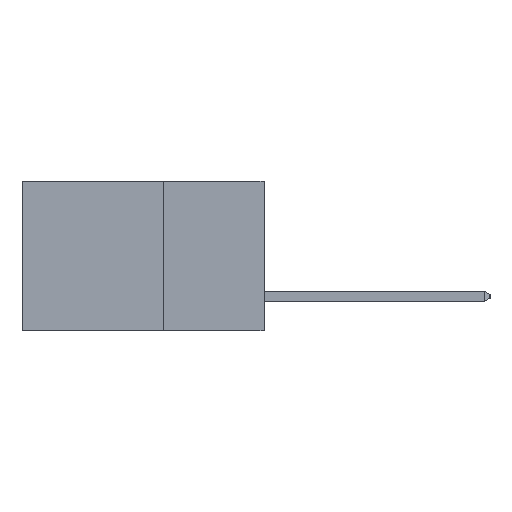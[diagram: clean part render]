
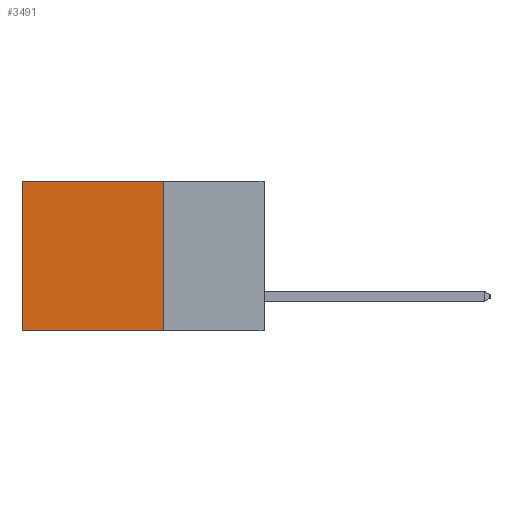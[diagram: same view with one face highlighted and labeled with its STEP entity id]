
A CAD part, left-side view. The second image highlights one B-rep face of the part: STEP entity #3491.
In plain terms, the highlighted planar face has unit normal (-1, 0, 0).
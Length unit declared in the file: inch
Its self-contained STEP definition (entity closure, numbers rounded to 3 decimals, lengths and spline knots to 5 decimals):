
#168 = EDGE_CURVE ( 'NONE', #5273, #9356, #3385, .T. ) ;
#925 = LINE ( 'NONE', #4226, #9724 ) ;
#1119 = DIRECTION ( 'NONE',  ( 0., 0., -1. ) ) ;
#1167 = DIRECTION ( 'NONE',  ( 1., 0., 0. ) ) ;
#1195 = CARTESIAN_POINT ( 'NONE',  ( 0.2615, 0.25, -0.37 ) ) ;
#1215 = PLANE ( 'NONE',  #4632 ) ;
#1447 = DIRECTION ( 'NONE',  ( 0., 1., 0. ) ) ;
#1473 = CARTESIAN_POINT ( 'NONE',  ( 0.2615, 0.25, -0.37 ) ) ;
#1525 = EDGE_CURVE ( 'NONE', #9356, #10380, #7017, .T. ) ;
#2842 = DIRECTION ( 'NONE',  ( 0., 1., 0. ) ) ;
#3385 = LINE ( 'NONE', #4524, #9996 ) ;
#3491 = ADVANCED_FACE ( 'NONE', ( #5857 ), #1215, .F. ) ;
#3927 = VECTOR ( 'NONE', #2842, 39.37008 ) ;
#4226 = CARTESIAN_POINT ( 'NONE',  ( 0.2615, 0.6, -0.37 ) ) ;
#4477 = VECTOR ( 'NONE', #1447, 39.37008 ) ;
#4524 = CARTESIAN_POINT ( 'NONE',  ( 0.2615, 0.25, -0.37 ) ) ;
#4539 = DIRECTION ( 'NONE',  ( 0., 0., -1. ) ) ;
#4632 = AXIS2_PLACEMENT_3D ( 'NONE', #1195, #1167, #1119 ) ;
#5273 = VERTEX_POINT ( 'NONE', #5674 ) ;
#5674 = CARTESIAN_POINT ( 'NONE',  ( 0.2615, 0.25, 0. ) ) ;
#5857 = FACE_OUTER_BOUND ( 'NONE', #10100, .T. ) ;
#6485 = ORIENTED_EDGE ( 'NONE', *, *, #9236, .T. ) ;
#6645 = ORIENTED_EDGE ( 'NONE', *, *, #8902, .T. ) ;
#6805 = DIRECTION ( 'NONE',  ( 0., 0., -1. ) ) ;
#7017 = LINE ( 'NONE', #1473, #4477 ) ;
#7164 = VERTEX_POINT ( 'NONE', #10984 ) ;
#7904 = LINE ( 'NONE', #8758, #3927 ) ;
#8631 = CARTESIAN_POINT ( 'NONE',  ( 0.2615, 0.6, -0.37 ) ) ;
#8758 = CARTESIAN_POINT ( 'NONE',  ( 0.2615, 0.25, 0. ) ) ;
#8902 = EDGE_CURVE ( 'NONE', #5273, #7164, #7904, .T. ) ;
#9236 = EDGE_CURVE ( 'NONE', #7164, #10380, #925, .T. ) ;
#9356 = VERTEX_POINT ( 'NONE', #10877 ) ;
#9718 = ORIENTED_EDGE ( 'NONE', *, *, #168, .F. ) ;
#9724 = VECTOR ( 'NONE', #6805, 39.37008 ) ;
#9996 = VECTOR ( 'NONE', #4539, 39.37008 ) ;
#10100 = EDGE_LOOP ( 'NONE', ( #6485, #10747, #9718, #6645 ) ) ;
#10380 = VERTEX_POINT ( 'NONE', #8631 ) ;
#10747 = ORIENTED_EDGE ( 'NONE', *, *, #1525, .F. ) ;
#10877 = CARTESIAN_POINT ( 'NONE',  ( 0.2615, 0.25, -0.37 ) ) ;
#10984 = CARTESIAN_POINT ( 'NONE',  ( 0.2615, 0.6, 0. ) ) ;
